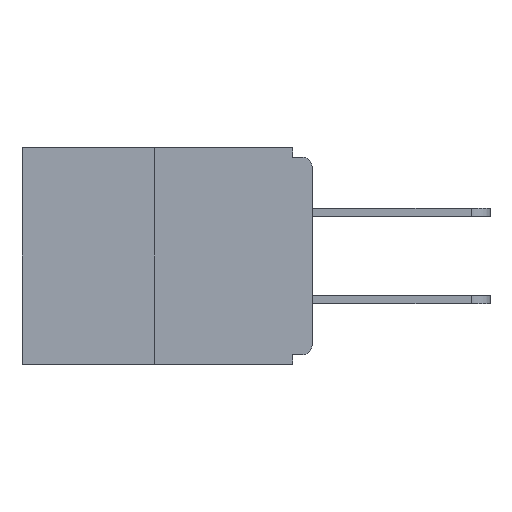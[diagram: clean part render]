
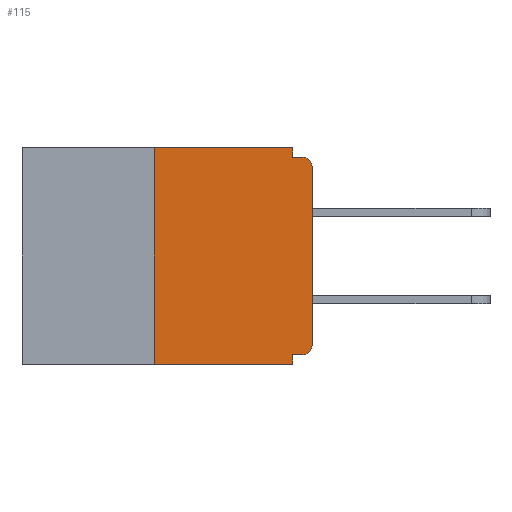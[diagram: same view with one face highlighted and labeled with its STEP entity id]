
A CAD part, left-side view. The second image highlights one B-rep face of the part: STEP entity #115.
In plain terms, the highlighted planar face has unit normal (-1, 0, 0).
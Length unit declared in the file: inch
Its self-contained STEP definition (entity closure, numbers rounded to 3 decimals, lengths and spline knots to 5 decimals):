
#25 = VERTEX_POINT ( 'NONE', #9137 ) ;
#115 = ADVANCED_FACE ( 'NONE', ( #8200 ), #1805, .F. ) ;
#673 = CARTESIAN_POINT ( 'NONE',  ( 0., 0.031, -0.343 ) ) ;
#812 = DIRECTION ( 'NONE',  ( 0., 0., -1. ) ) ;
#1199 = CARTESIAN_POINT ( 'NONE',  ( 0., 0., -0.328 ) ) ;
#1258 = CARTESIAN_POINT ( 'NONE',  ( 0., 0., 0. ) ) ;
#1348 = LINE ( 'NONE', #9289, #6328 ) ;
#1758 = VECTOR ( 'NONE', #6833, 39.37008 ) ;
#1804 = VERTEX_POINT ( 'NONE', #8635 ) ;
#1805 = PLANE ( 'NONE',  #5388 ) ;
#1956 = EDGE_CURVE ( 'NONE', #3984, #9696, #7280, .T. ) ;
#2040 = VECTOR ( 'NONE', #9884, 39.37008 ) ;
#2339 = LINE ( 'NONE', #8892, #2040 ) ;
#2560 = CARTESIAN_POINT ( 'NONE',  ( 0., 0.25, -0.343 ) ) ;
#2741 = ORIENTED_EDGE ( 'NONE', *, *, #7531, .T. ) ;
#2918 = LINE ( 'NONE', #9719, #1758 ) ;
#2988 = ORIENTED_EDGE ( 'NONE', *, *, #5287, .F. ) ;
#3094 = ORIENTED_EDGE ( 'NONE', *, *, #6755, .T. ) ;
#3117 = ORIENTED_EDGE ( 'NONE', *, *, #5135, .T. ) ;
#3363 = VECTOR ( 'NONE', #3514, 39.37008 ) ;
#3404 = CARTESIAN_POINT ( 'NONE',  ( 0., 0.25, 0. ) ) ;
#3439 = VECTOR ( 'NONE', #11535, 39.37008 ) ;
#3470 = CARTESIAN_POINT ( 'NONE',  ( 0., 0.46, -0.343 ) ) ;
#3514 = DIRECTION ( 'NONE',  ( 0., -1., 0. ) ) ;
#3589 = DIRECTION ( 'NONE',  ( 0., 0., -1. ) ) ;
#3850 = DIRECTION ( 'NONE',  ( -1., 0., 0. ) ) ;
#3951 = VERTEX_POINT ( 'NONE', #11664 ) ;
#3984 = VERTEX_POINT ( 'NONE', #10264 ) ;
#4050 = DIRECTION ( 'NONE',  ( -1., 0., 0. ) ) ;
#4138 = VERTEX_POINT ( 'NONE', #5117 ) ;
#4162 = LINE ( 'NONE', #1199, #3439 ) ;
#4351 = VERTEX_POINT ( 'NONE', #4571 ) ;
#4424 = CARTESIAN_POINT ( 'NONE',  ( 0., 0.031, -0.328 ) ) ;
#4571 = CARTESIAN_POINT ( 'NONE',  ( 0., 0., -0.313 ) ) ;
#4581 = EDGE_CURVE ( 'NONE', #1804, #25, #2918, .T. ) ;
#4858 = CARTESIAN_POINT ( 'NONE',  ( 0., 0.015, -0.313 ) ) ;
#4948 = DIRECTION ( 'NONE',  ( 0., -1., 0. ) ) ;
#5117 = CARTESIAN_POINT ( 'NONE',  ( 0., 0.015, -0.328 ) ) ;
#5135 = EDGE_CURVE ( 'NONE', #3951, #9696, #10387, .T. ) ;
#5287 = EDGE_CURVE ( 'NONE', #9814, #9892, #2339, .T. ) ;
#5388 = AXIS2_PLACEMENT_3D ( 'NONE', #6384, #11193, #3589 ) ;
#5703 = ORIENTED_EDGE ( 'NONE', *, *, #8314, .F. ) ;
#5790 = DIRECTION ( 'NONE',  ( 0., 0., -1. ) ) ;
#5947 = DIRECTION ( 'NONE',  ( 0., 0., -1. ) ) ;
#6285 = VERTEX_POINT ( 'NONE', #2560 ) ;
#6328 = VECTOR ( 'NONE', #812, 39.37008 ) ;
#6384 = CARTESIAN_POINT ( 'NONE',  ( 0., 0.46, 0. ) ) ;
#6446 = EDGE_CURVE ( 'NONE', #6285, #1804, #11555, .T. ) ;
#6504 = VECTOR ( 'NONE', #6987, 39.37008 ) ;
#6755 = EDGE_CURVE ( 'NONE', #4138, #4351, #10193, .T. ) ;
#6833 = DIRECTION ( 'NONE',  ( 0., -1., 0. ) ) ;
#6987 = DIRECTION ( 'NONE',  ( 0., 0., 1. ) ) ;
#7039 = EDGE_LOOP ( 'NONE', ( #9468, #8493, #9255, #2988, #5703, #3094, #2741, #3117, #10883, #10318 ) ) ;
#7230 = DIRECTION ( 'NONE',  ( 0., 0., 1. ) ) ;
#7280 = LINE ( 'NONE', #9729, #10788 ) ;
#7296 = VECTOR ( 'NONE', #7230, 39.37008 ) ;
#7531 = EDGE_CURVE ( 'NONE', #4351, #3951, #11676, .T. ) ;
#7758 = AXIS2_PLACEMENT_3D ( 'NONE', #4858, #4050, #5790 ) ;
#8200 = FACE_OUTER_BOUND ( 'NONE', #7039, .T. ) ;
#8314 = EDGE_CURVE ( 'NONE', #4138, #9814, #4162, .T. ) ;
#8493 = ORIENTED_EDGE ( 'NONE', *, *, #6446, .F. ) ;
#8635 = CARTESIAN_POINT ( 'NONE',  ( 0., 0.25, 0. ) ) ;
#8892 = CARTESIAN_POINT ( 'NONE',  ( 0., 0.031, -0.343 ) ) ;
#9137 = CARTESIAN_POINT ( 'NONE',  ( 0., 0.031, 0. ) ) ;
#9226 = EDGE_CURVE ( 'NONE', #25, #3984, #1348, .T. ) ;
#9255 = ORIENTED_EDGE ( 'NONE', *, *, #10550, .T. ) ;
#9289 = CARTESIAN_POINT ( 'NONE',  ( 0., 0.031, 0. ) ) ;
#9468 = ORIENTED_EDGE ( 'NONE', *, *, #4581, .F. ) ;
#9696 = VERTEX_POINT ( 'NONE', #10767 ) ;
#9719 = CARTESIAN_POINT ( 'NONE',  ( 0., 0.46, 0. ) ) ;
#9729 = CARTESIAN_POINT ( 'NONE',  ( 0., 0., -0.015 ) ) ;
#9814 = VERTEX_POINT ( 'NONE', #4424 ) ;
#9884 = DIRECTION ( 'NONE',  ( 0., 0., -1. ) ) ;
#9892 = VERTEX_POINT ( 'NONE', #673 ) ;
#10193 = CIRCLE ( 'NONE', #7758, 0.015 ) ;
#10264 = CARTESIAN_POINT ( 'NONE',  ( 0., 0.031, -0.015 ) ) ;
#10296 = CARTESIAN_POINT ( 'NONE',  ( 0., 0.015, -0.03 ) ) ;
#10318 = ORIENTED_EDGE ( 'NONE', *, *, #9226, .F. ) ;
#10387 = CIRCLE ( 'NONE', #11659, 0.015 ) ;
#10550 = EDGE_CURVE ( 'NONE', #6285, #9892, #10679, .T. ) ;
#10679 = LINE ( 'NONE', #3470, #3363 ) ;
#10767 = CARTESIAN_POINT ( 'NONE',  ( 0., 0.015, -0.015 ) ) ;
#10788 = VECTOR ( 'NONE', #4948, 39.37008 ) ;
#10883 = ORIENTED_EDGE ( 'NONE', *, *, #1956, .F. ) ;
#11193 = DIRECTION ( 'NONE',  ( 1., 0., 0. ) ) ;
#11535 = DIRECTION ( 'NONE',  ( 0., 1., 0. ) ) ;
#11555 = LINE ( 'NONE', #3404, #7296 ) ;
#11659 = AXIS2_PLACEMENT_3D ( 'NONE', #10296, #3850, #5947 ) ;
#11664 = CARTESIAN_POINT ( 'NONE',  ( 0., 0., -0.03 ) ) ;
#11676 = LINE ( 'NONE', #1258, #6504 ) ;
